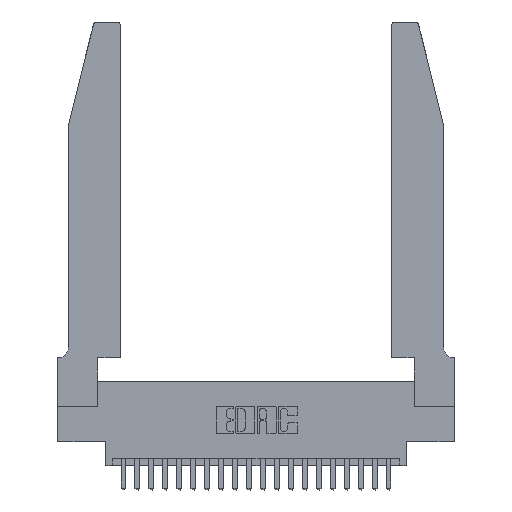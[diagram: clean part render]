
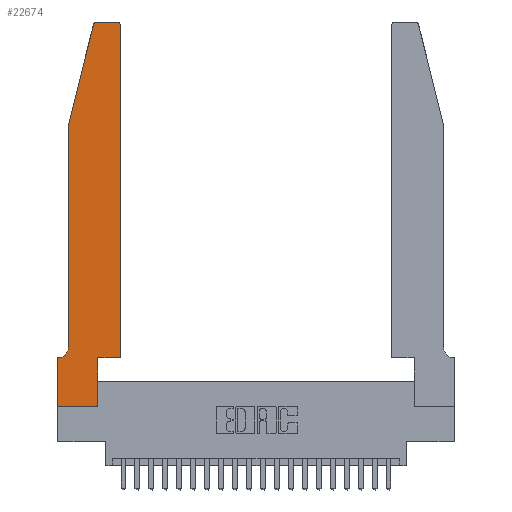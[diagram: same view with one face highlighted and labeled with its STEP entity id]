
A CAD part, top view. The second image highlights one B-rep face of the part: STEP entity #22674.
In plain terms, the highlighted planar face has unit normal (0, 0, 1).
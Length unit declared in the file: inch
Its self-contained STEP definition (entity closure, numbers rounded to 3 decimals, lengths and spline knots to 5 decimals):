
#157 = CARTESIAN_POINT ( 'NONE',  ( 0.25487, 2.72718, 0.37 ) ) ;
#707 = EDGE_CURVE ( 'NONE', #1813, #18288, #7178, .T. ) ;
#728 = CARTESIAN_POINT ( 'NONE',  ( 0.0055, 0.42, 0.37 ) ) ;
#759 = VECTOR ( 'NONE', #15653, 39.37008 ) ;
#1136 = LINE ( 'NONE', #4178, #20014 ) ;
#1747 = ORIENTED_EDGE ( 'NONE', *, *, #4541, .T. ) ;
#1813 = VERTEX_POINT ( 'NONE', #5442 ) ;
#2087 = VECTOR ( 'NONE', #8060, 39.37008 ) ;
#2507 = CIRCLE ( 'NONE', #23475, 0.03 ) ;
#2593 = DIRECTION ( 'NONE',  ( -1., 0., 0. ) ) ;
#2699 = ORIENTED_EDGE ( 'NONE', *, *, #15369, .T. ) ;
#3183 = CARTESIAN_POINT ( 'NONE',  ( 0.2865, 0., 0.37 ) ) ;
#3624 = EDGE_CURVE ( 'NONE', #21070, #16744, #11338, .T. ) ;
#3818 = CARTESIAN_POINT ( 'NONE',  ( 0.4205, 2.75, 0.37 ) ) ;
#3859 = VECTOR ( 'NONE', #10163, 39.37008 ) ;
#4178 = CARTESIAN_POINT ( 'NONE',  ( 0.0755, 0.35, 0.37 ) ) ;
#4541 = EDGE_CURVE ( 'NONE', #6146, #5963, #7328, .T. ) ;
#4562 = EDGE_CURVE ( 'NONE', #14743, #5635, #15848, .T. ) ;
#4637 = CARTESIAN_POINT ( 'NONE',  ( 0.4505, 0.35, 0.37 ) ) ;
#4962 = EDGE_CURVE ( 'NONE', #16744, #17875, #22392, .T. ) ;
#5216 = EDGE_CURVE ( 'NONE', #17875, #14341, #8708, .T. ) ;
#5442 = CARTESIAN_POINT ( 'NONE',  ( 0., 0.35, 0.37 ) ) ;
#5447 = AXIS2_PLACEMENT_3D ( 'NONE', #14057, #6785, #19552 ) ;
#5538 = CARTESIAN_POINT ( 'NONE',  ( 0.4505, 0.35, 0.37 ) ) ;
#5635 = VERTEX_POINT ( 'NONE', #5909 ) ;
#5909 = CARTESIAN_POINT ( 'NONE',  ( 0.284, 2.75, 0.37 ) ) ;
#5962 = DIRECTION ( 'NONE',  ( 0., 0., 1. ) ) ;
#5963 = VERTEX_POINT ( 'NONE', #14036 ) ;
#6115 = VECTOR ( 'NONE', #22185, 39.37008 ) ;
#6146 = VERTEX_POINT ( 'NONE', #19999 ) ;
#6357 = CIRCLE ( 'NONE', #20943, 0.03 ) ;
#6641 = ORIENTED_EDGE ( 'NONE', *, *, #4562, .T. ) ;
#6785 = DIRECTION ( 'NONE',  ( 0., 0., 1. ) ) ;
#6957 = LINE ( 'NONE', #19013, #2087 ) ;
#7178 = LINE ( 'NONE', #19744, #21123 ) ;
#7328 = CIRCLE ( 'NONE', #20911, 0.07 ) ;
#7353 = ORIENTED_EDGE ( 'NONE', *, *, #16815, .T. ) ;
#7515 = ORIENTED_EDGE ( 'NONE', *, *, #5216, .T. ) ;
#7927 = DIRECTION ( 'NONE',  ( -1., 0., 0. ) ) ;
#8060 = DIRECTION ( 'NONE',  ( 1., 0., 0. ) ) ;
#8215 = DIRECTION ( 'NONE',  ( 0., 0., 1. ) ) ;
#8549 = PLANE ( 'NONE',  #5447 ) ;
#8708 = LINE ( 'NONE', #4637, #3859 ) ;
#9556 = ORIENTED_EDGE ( 'NONE', *, *, #3624, .T. ) ;
#9954 = DIRECTION ( 'NONE',  ( -1., 0., 0. ) ) ;
#9979 = ORIENTED_EDGE ( 'NONE', *, *, #17995, .T. ) ;
#10163 = DIRECTION ( 'NONE',  ( 0., 1., 0. ) ) ;
#10305 = ORIENTED_EDGE ( 'NONE', *, *, #4962, .T. ) ;
#10794 = ORIENTED_EDGE ( 'NONE', *, *, #13167, .T. ) ;
#11002 = LINE ( 'NONE', #12811, #6115 ) ;
#11056 = VECTOR ( 'NONE', #9954, 39.37008 ) ;
#11115 = LINE ( 'NONE', #13846, #759 ) ;
#11220 = CARTESIAN_POINT ( 'NONE',  ( 0.2865, 0.35, 0.37 ) ) ;
#11265 = ORIENTED_EDGE ( 'NONE', *, *, #20443, .T. ) ;
#11338 = LINE ( 'NONE', #11220, #20992 ) ;
#12721 = VECTOR ( 'NONE', #16537, 39.37008 ) ;
#12811 = CARTESIAN_POINT ( 'NONE',  ( 0.0755, 2., 0.37 ) ) ;
#13088 = EDGE_CURVE ( 'NONE', #5635, #18958, #2507, .T. ) ;
#13167 = EDGE_CURVE ( 'NONE', #16105, #6146, #11115, .T. ) ;
#13427 = FACE_OUTER_BOUND ( 'NONE', #19937, .T. ) ;
#13529 = DIRECTION ( 'NONE',  ( 0., 0., -1. ) ) ;
#13846 = CARTESIAN_POINT ( 'NONE',  ( 0.0755, 2., 0.37 ) ) ;
#14027 = ORIENTED_EDGE ( 'NONE', *, *, #13088, .T. ) ;
#14036 = CARTESIAN_POINT ( 'NONE',  ( 0.0055, 0.35, 0.37 ) ) ;
#14057 = CARTESIAN_POINT ( 'NONE',  ( 0., 0.35, 0.37 ) ) ;
#14130 = CARTESIAN_POINT ( 'NONE',  ( 0., 0., 0.37 ) ) ;
#14341 = VERTEX_POINT ( 'NONE', #19151 ) ;
#14743 = VERTEX_POINT ( 'NONE', #3818 ) ;
#15296 = CARTESIAN_POINT ( 'NONE',  ( 0.2865, 0.35, 0.37 ) ) ;
#15369 = EDGE_CURVE ( 'NONE', #18958, #16105, #11002, .T. ) ;
#15653 = DIRECTION ( 'NONE',  ( 0., -1., 0. ) ) ;
#15848 = LINE ( 'NONE', #17190, #11056 ) ;
#16105 = VERTEX_POINT ( 'NONE', #21987 ) ;
#16537 = DIRECTION ( 'NONE',  ( 1., 0., 0. ) ) ;
#16744 = VERTEX_POINT ( 'NONE', #15296 ) ;
#16815 = EDGE_CURVE ( 'NONE', #14341, #14743, #6357, .T. ) ;
#16885 = CARTESIAN_POINT ( 'NONE',  ( 0.284, 2.72, 0.37 ) ) ;
#17190 = CARTESIAN_POINT ( 'NONE',  ( 0.2605, 2.75, 0.37 ) ) ;
#17595 = ORIENTED_EDGE ( 'NONE', *, *, #707, .T. ) ;
#17875 = VERTEX_POINT ( 'NONE', #5538 ) ;
#17995 = EDGE_CURVE ( 'NONE', #5963, #1813, #1136, .T. ) ;
#18288 = VERTEX_POINT ( 'NONE', #14130 ) ;
#18546 = DIRECTION ( 'NONE',  ( 0., 1., 0. ) ) ;
#18744 = DIRECTION ( 'NONE',  ( 1., 0., 0. ) ) ;
#18958 = VERTEX_POINT ( 'NONE', #157 ) ;
#19013 = CARTESIAN_POINT ( 'NONE',  ( 0., 0., 0.37 ) ) ;
#19151 = CARTESIAN_POINT ( 'NONE',  ( 0.4505, 2.72, 0.37 ) ) ;
#19153 = CARTESIAN_POINT ( 'NONE',  ( 0.4205, 2.72, 0.37 ) ) ;
#19416 = CARTESIAN_POINT ( 'NONE',  ( 0.4505, 0.35, 0.37 ) ) ;
#19552 = DIRECTION ( 'NONE',  ( 1., 0., 0. ) ) ;
#19744 = CARTESIAN_POINT ( 'NONE',  ( 0., 0., 0.37 ) ) ;
#19937 = EDGE_LOOP ( 'NONE', ( #6641, #14027, #2699, #10794, #1747, #9979, #17595, #11265, #9556, #10305, #7515, #7353 ) ) ;
#19999 = CARTESIAN_POINT ( 'NONE',  ( 0.0755, 0.42, 0.37 ) ) ;
#20014 = VECTOR ( 'NONE', #7927, 39.37008 ) ;
#20114 = DIRECTION ( 'NONE',  ( 0., -1., 0. ) ) ;
#20443 = EDGE_CURVE ( 'NONE', #18288, #21070, #6957, .T. ) ;
#20911 = AXIS2_PLACEMENT_3D ( 'NONE', #728, #13529, #2593 ) ;
#20943 = AXIS2_PLACEMENT_3D ( 'NONE', #19153, #8215, #20950 ) ;
#20950 = DIRECTION ( 'NONE',  ( 1., 0., 0. ) ) ;
#20992 = VECTOR ( 'NONE', #18546, 39.37008 ) ;
#21070 = VERTEX_POINT ( 'NONE', #3183 ) ;
#21123 = VECTOR ( 'NONE', #20114, 39.37008 ) ;
#21987 = CARTESIAN_POINT ( 'NONE',  ( 0.0755, 2., 0.37 ) ) ;
#22185 = DIRECTION ( 'NONE',  ( -0.239, -0.971, 0. ) ) ;
#22392 = LINE ( 'NONE', #19416, #12721 ) ;
#22674 = ADVANCED_FACE ( 'NONE', ( #13427 ), #8549, .T. ) ;
#23475 = AXIS2_PLACEMENT_3D ( 'NONE', #16885, #5962, #18744 ) ;
